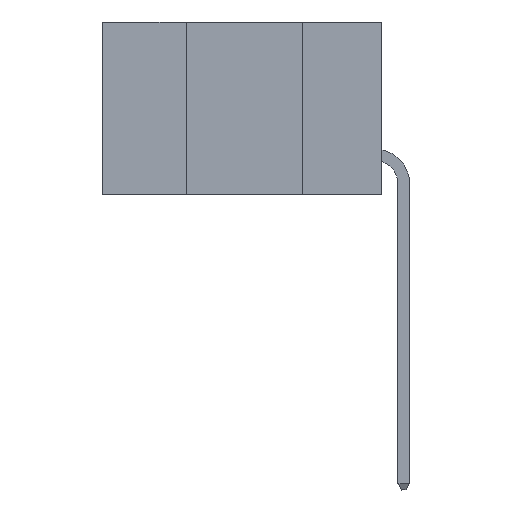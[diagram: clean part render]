
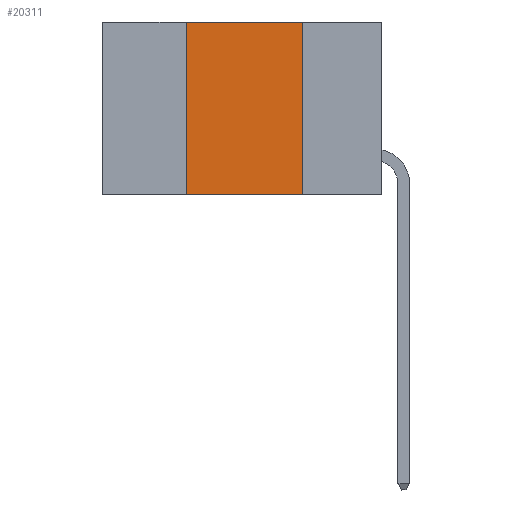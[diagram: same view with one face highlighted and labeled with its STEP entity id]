
A CAD part, left-side view. The second image highlights one B-rep face of the part: STEP entity #20311.
In plain terms, the highlighted planar face has unit normal (-1, 0, 0).
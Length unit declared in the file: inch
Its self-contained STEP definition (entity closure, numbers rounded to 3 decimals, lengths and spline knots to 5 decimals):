
#25 = ORIENTED_EDGE ( 'NONE', *, *, #549, .F. ) ;
#549 = EDGE_CURVE ( 'NONE', #22702, #9166, #15563, .T. ) ;
#863 = ORIENTED_EDGE ( 'NONE', *, *, #1477, .F. ) ;
#1477 = EDGE_CURVE ( 'NONE', #14651, #4925, #2553, .T. ) ;
#2553 = LINE ( 'NONE', #11344, #12748 ) ;
#3070 = DIRECTION ( 'NONE',  ( 1., 0., 0. ) ) ;
#4346 = EDGE_CURVE ( 'NONE', #14651, #9166, #16709, .T. ) ;
#4437 = CARTESIAN_POINT ( 'NONE',  ( 0., 0.17, 0. ) ) ;
#4925 = VERTEX_POINT ( 'NONE', #23720 ) ;
#7034 = FACE_OUTER_BOUND ( 'NONE', #22354, .T. ) ;
#7126 = PLANE ( 'NONE',  #8338 ) ;
#7251 = ORIENTED_EDGE ( 'NONE', *, *, #7601, .F. ) ;
#7601 = EDGE_CURVE ( 'NONE', #4925, #22702, #20567, .T. ) ;
#8338 = AXIS2_PLACEMENT_3D ( 'NONE', #16633, #3070, #16976 ) ;
#9166 = VERTEX_POINT ( 'NONE', #11227 ) ;
#11227 = CARTESIAN_POINT ( 'NONE',  ( 0., 0.17, -0.37 ) ) ;
#11344 = CARTESIAN_POINT ( 'NONE',  ( 0., 0.42, 0. ) ) ;
#12748 = VECTOR ( 'NONE', #21598, 39.37008 ) ;
#12970 = VECTOR ( 'NONE', #20328, 39.37008 ) ;
#13145 = CARTESIAN_POINT ( 'NONE',  ( 0., 0.6, 0. ) ) ;
#14651 = VERTEX_POINT ( 'NONE', #15540 ) ;
#15540 = CARTESIAN_POINT ( 'NONE',  ( 0., 0.42, -0.37 ) ) ;
#15563 = LINE ( 'NONE', #4437, #25455 ) ;
#16633 = CARTESIAN_POINT ( 'NONE',  ( 0., 0.6, 0. ) ) ;
#16709 = LINE ( 'NONE', #16815, #12970 ) ;
#16815 = CARTESIAN_POINT ( 'NONE',  ( 0., 0.6, -0.37 ) ) ;
#16976 = DIRECTION ( 'NONE',  ( 0., 0., -1. ) ) ;
#17376 = DIRECTION ( 'NONE',  ( 0., -1., 0. ) ) ;
#18210 = DIRECTION ( 'NONE',  ( 0., 0., -1. ) ) ;
#19851 = CARTESIAN_POINT ( 'NONE',  ( 0., 0.17, 0. ) ) ;
#20230 = ORIENTED_EDGE ( 'NONE', *, *, #4346, .T. ) ;
#20311 = ADVANCED_FACE ( 'NONE', ( #7034 ), #7126, .F. ) ;
#20328 = DIRECTION ( 'NONE',  ( 0., -1., 0. ) ) ;
#20567 = LINE ( 'NONE', #13145, #25206 ) ;
#21598 = DIRECTION ( 'NONE',  ( 0., 0., 1. ) ) ;
#22354 = EDGE_LOOP ( 'NONE', ( #25, #7251, #863, #20230 ) ) ;
#22702 = VERTEX_POINT ( 'NONE', #19851 ) ;
#23720 = CARTESIAN_POINT ( 'NONE',  ( 0., 0.42, 0. ) ) ;
#25206 = VECTOR ( 'NONE', #17376, 39.37008 ) ;
#25455 = VECTOR ( 'NONE', #18210, 39.37008 ) ;
